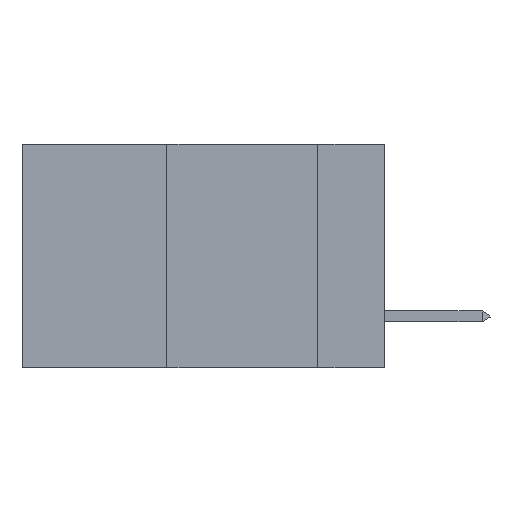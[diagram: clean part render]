
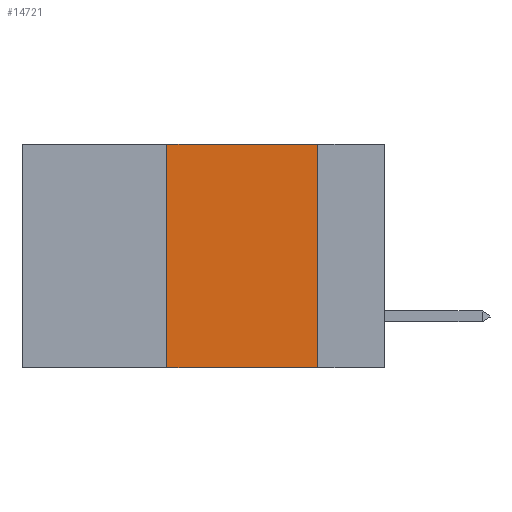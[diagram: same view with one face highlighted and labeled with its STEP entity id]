
A CAD part, left-side view. The second image highlights one B-rep face of the part: STEP entity #14721.
In plain terms, the highlighted planar face has unit normal (-1, 0, 0).
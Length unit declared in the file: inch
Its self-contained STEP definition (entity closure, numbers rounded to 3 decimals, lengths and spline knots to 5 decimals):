
#339 = DIRECTION ( 'NONE',  ( 0., 0., -1. ) ) ;
#753 = FACE_OUTER_BOUND ( 'NONE', #37406, .T. ) ;
#2556 = CARTESIAN_POINT ( 'NONE',  ( 0., 0.36, -0.37 ) ) ;
#2564 = CARTESIAN_POINT ( 'NONE',  ( 0., 0.6, 0. ) ) ;
#3190 = DIRECTION ( 'NONE',  ( 1., 0., 0. ) ) ;
#5002 = ORIENTED_EDGE ( 'NONE', *, *, #33799, .F. ) ;
#7993 = ORIENTED_EDGE ( 'NONE', *, *, #37148, .F. ) ;
#9737 = LINE ( 'NONE', #2564, #18526 ) ;
#14658 = VERTEX_POINT ( 'NONE', #23928 ) ;
#14721 = ADVANCED_FACE ( 'NONE', ( #753 ), #31738, .F. ) ;
#14813 = VECTOR ( 'NONE', #29210, 39.37008 ) ;
#16119 = CARTESIAN_POINT ( 'NONE',  ( 0., 0.11, 0. ) ) ;
#16483 = VECTOR ( 'NONE', #22213, 39.37008 ) ;
#16856 = ORIENTED_EDGE ( 'NONE', *, *, #26774, .T. ) ;
#18526 = VECTOR ( 'NONE', #20689, 39.37008 ) ;
#20227 = CARTESIAN_POINT ( 'NONE',  ( 0., 0.6, 0. ) ) ;
#20410 = DIRECTION ( 'NONE',  ( 0., 0., 1. ) ) ;
#20689 = DIRECTION ( 'NONE',  ( 0., -1., 0. ) ) ;
#22213 = DIRECTION ( 'NONE',  ( 0., 0., -1. ) ) ;
#23928 = CARTESIAN_POINT ( 'NONE',  ( 0., 0.36, 0. ) ) ;
#25004 = VERTEX_POINT ( 'NONE', #16119 ) ;
#26774 = EDGE_CURVE ( 'NONE', #32139, #33942, #34546, .T. ) ;
#29075 = AXIS2_PLACEMENT_3D ( 'NONE', #20227, #3190, #339 ) ;
#29210 = DIRECTION ( 'NONE',  ( 0., -1., 0. ) ) ;
#29243 = EDGE_CURVE ( 'NONE', #32139, #14658, #30195, .T. ) ;
#29459 = CARTESIAN_POINT ( 'NONE',  ( 0., 0.6, -0.37 ) ) ;
#30195 = LINE ( 'NONE', #37936, #32050 ) ;
#31738 = PLANE ( 'NONE',  #29075 ) ;
#32050 = VECTOR ( 'NONE', #20410, 39.37008 ) ;
#32139 = VERTEX_POINT ( 'NONE', #2556 ) ;
#33799 = EDGE_CURVE ( 'NONE', #25004, #33942, #34841, .T. ) ;
#33816 = ORIENTED_EDGE ( 'NONE', *, *, #29243, .F. ) ;
#33942 = VERTEX_POINT ( 'NONE', #34378 ) ;
#34378 = CARTESIAN_POINT ( 'NONE',  ( 0., 0.11, -0.37 ) ) ;
#34546 = LINE ( 'NONE', #29459, #14813 ) ;
#34841 = LINE ( 'NONE', #37163, #16483 ) ;
#37148 = EDGE_CURVE ( 'NONE', #14658, #25004, #9737, .T. ) ;
#37163 = CARTESIAN_POINT ( 'NONE',  ( 0., 0.11, 0. ) ) ;
#37406 = EDGE_LOOP ( 'NONE', ( #5002, #7993, #33816, #16856 ) ) ;
#37936 = CARTESIAN_POINT ( 'NONE',  ( 0., 0.36, 0. ) ) ;
